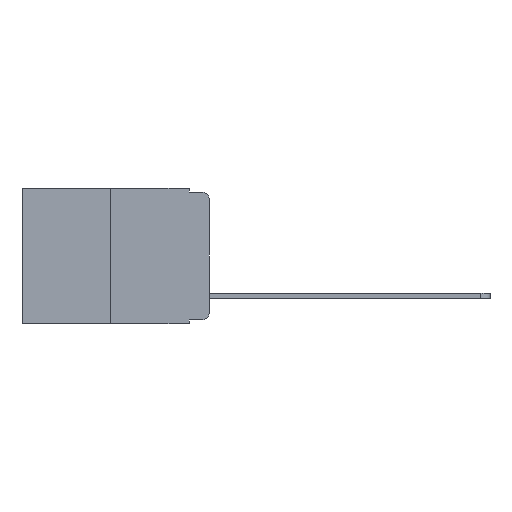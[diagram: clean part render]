
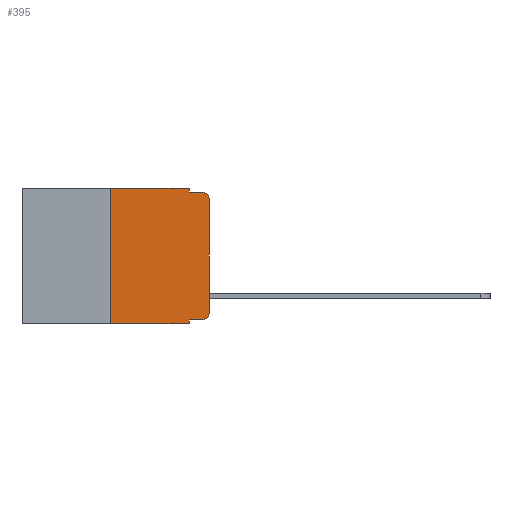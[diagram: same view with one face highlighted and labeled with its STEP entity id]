
A CAD part, left-side view. The second image highlights one B-rep face of the part: STEP entity #395.
In plain terms, the highlighted planar face has unit normal (-1, 0, 0).
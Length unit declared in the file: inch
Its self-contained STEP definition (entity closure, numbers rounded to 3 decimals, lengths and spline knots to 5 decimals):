
#41 = VERTEX_POINT ( 'NONE', #4234 ) ;
#271 = EDGE_CURVE ( 'NONE', #1706, #6711, #9293, .T. ) ;
#337 = VERTEX_POINT ( 'NONE', #8709 ) ;
#395 = ADVANCED_FACE ( 'NONE', ( #1490 ), #6747, .F. ) ;
#448 = VECTOR ( 'NONE', #8648, 39.37008 ) ;
#515 = DIRECTION ( 'NONE',  ( 0., -1., 0. ) ) ;
#679 = ORIENTED_EDGE ( 'NONE', *, *, #7900, .F. ) ;
#728 = LINE ( 'NONE', #1204, #448 ) ;
#745 = VECTOR ( 'NONE', #4934, 39.37008 ) ;
#969 = ORIENTED_EDGE ( 'NONE', *, *, #10487, .T. ) ;
#1012 = CARTESIAN_POINT ( 'NONE',  ( 0., 0.02, -0.333 ) ) ;
#1031 = EDGE_LOOP ( 'NONE', ( #1630, #4977, #679, #3099, #3904, #8712, #969, #8114, #4585, #9305 ) ) ;
#1162 = CARTESIAN_POINT ( 'NONE',  ( 0., 0., -0.313 ) ) ;
#1204 = CARTESIAN_POINT ( 'NONE',  ( 0., 0.051, -0.01 ) ) ;
#1225 = AXIS2_PLACEMENT_3D ( 'NONE', #5626, #6207, #6199 ) ;
#1490 = FACE_OUTER_BOUND ( 'NONE', #1031, .T. ) ;
#1497 = LINE ( 'NONE', #6130, #9902 ) ;
#1523 = EDGE_CURVE ( 'NONE', #337, #6897, #10321, .T. ) ;
#1630 = ORIENTED_EDGE ( 'NONE', *, *, #271, .T. ) ;
#1706 = VERTEX_POINT ( 'NONE', #1162 ) ;
#1831 = VERTEX_POINT ( 'NONE', #6097 ) ;
#1940 = VERTEX_POINT ( 'NONE', #7417 ) ;
#2019 = EDGE_CURVE ( 'NONE', #6711, #41, #8284, .T. ) ;
#2020 = EDGE_CURVE ( 'NONE', #2855, #1706, #10310, .T. ) ;
#2799 = DIRECTION ( 'NONE',  ( 0., -1., 0. ) ) ;
#2855 = VERTEX_POINT ( 'NONE', #1012 ) ;
#2981 = EDGE_CURVE ( 'NONE', #6897, #1940, #7904, .T. ) ;
#3023 = LINE ( 'NONE', #10417, #745 ) ;
#3099 = ORIENTED_EDGE ( 'NONE', *, *, #5181, .F. ) ;
#3163 = CARTESIAN_POINT ( 'NONE',  ( 0., 0.051, -0.01 ) ) ;
#3527 = AXIS2_PLACEMENT_3D ( 'NONE', #3577, #4171, #7919 ) ;
#3577 = CARTESIAN_POINT ( 'NONE',  ( 0., 0.02, -0.03 ) ) ;
#3611 = CARTESIAN_POINT ( 'NONE',  ( 0., 0.473, 0. ) ) ;
#3904 = ORIENTED_EDGE ( 'NONE', *, *, #2981, .F. ) ;
#3983 = VECTOR ( 'NONE', #7797, 39.37008 ) ;
#4027 = VECTOR ( 'NONE', #2799, 39.37008 ) ;
#4171 = DIRECTION ( 'NONE',  ( -1., 0., 0. ) ) ;
#4234 = CARTESIAN_POINT ( 'NONE',  ( 0., 0.02, -0.01 ) ) ;
#4266 = DIRECTION ( 'NONE',  ( 0., -1., 0. ) ) ;
#4585 = ORIENTED_EDGE ( 'NONE', *, *, #5970, .T. ) ;
#4663 = AXIS2_PLACEMENT_3D ( 'NONE', #7662, #8071, #6866 ) ;
#4756 = CARTESIAN_POINT ( 'NONE',  ( 0., 0.051, -0.333 ) ) ;
#4934 = DIRECTION ( 'NONE',  ( 0., 0., -1. ) ) ;
#4977 = ORIENTED_EDGE ( 'NONE', *, *, #2019, .T. ) ;
#5181 = EDGE_CURVE ( 'NONE', #1940, #9595, #1497, .T. ) ;
#5460 = DIRECTION ( 'NONE',  ( 0., 0., -1. ) ) ;
#5626 = CARTESIAN_POINT ( 'NONE',  ( 0., 0.473, 0. ) ) ;
#5808 = VECTOR ( 'NONE', #515, 39.37008 ) ;
#5970 = EDGE_CURVE ( 'NONE', #6853, #2855, #6730, .T. ) ;
#6097 = CARTESIAN_POINT ( 'NONE',  ( 0., 0.051, -0.343 ) ) ;
#6130 = CARTESIAN_POINT ( 'NONE',  ( 0., 0.051, 0. ) ) ;
#6199 = DIRECTION ( 'NONE',  ( 0., 0., -1. ) ) ;
#6207 = DIRECTION ( 'NONE',  ( 1., 0., 0. ) ) ;
#6240 = LINE ( 'NONE', #10011, #4027 ) ;
#6711 = VERTEX_POINT ( 'NONE', #7780 ) ;
#6730 = LINE ( 'NONE', #9470, #10590 ) ;
#6747 = PLANE ( 'NONE',  #1225 ) ;
#6853 = VERTEX_POINT ( 'NONE', #4756 ) ;
#6866 = DIRECTION ( 'NONE',  ( 0., 0., -1. ) ) ;
#6897 = VERTEX_POINT ( 'NONE', #8162 ) ;
#7417 = CARTESIAN_POINT ( 'NONE',  ( 0., 0.051, 0. ) ) ;
#7459 = EDGE_CURVE ( 'NONE', #6853, #1831, #3023, .T. ) ;
#7662 = CARTESIAN_POINT ( 'NONE',  ( 0., 0.02, -0.313 ) ) ;
#7780 = CARTESIAN_POINT ( 'NONE',  ( 0., 0., -0.03 ) ) ;
#7797 = DIRECTION ( 'NONE',  ( 0., 0., 1. ) ) ;
#7900 = EDGE_CURVE ( 'NONE', #9595, #41, #728, .T. ) ;
#7904 = LINE ( 'NONE', #3611, #5808 ) ;
#7919 = DIRECTION ( 'NONE',  ( 0., 0., -1. ) ) ;
#7931 = CARTESIAN_POINT ( 'NONE',  ( 0., 0., 0. ) ) ;
#7943 = DIRECTION ( 'NONE',  ( 0., 0., 1. ) ) ;
#8071 = DIRECTION ( 'NONE',  ( -1., 0., 0. ) ) ;
#8114 = ORIENTED_EDGE ( 'NONE', *, *, #7459, .F. ) ;
#8162 = CARTESIAN_POINT ( 'NONE',  ( 0., 0.25, 0. ) ) ;
#8284 = CIRCLE ( 'NONE', #3527, 0.02 ) ;
#8648 = DIRECTION ( 'NONE',  ( 0., -1., 0. ) ) ;
#8709 = CARTESIAN_POINT ( 'NONE',  ( 0., 0.25, -0.343 ) ) ;
#8712 = ORIENTED_EDGE ( 'NONE', *, *, #1523, .F. ) ;
#8828 = VECTOR ( 'NONE', #7943, 39.37008 ) ;
#9293 = LINE ( 'NONE', #7931, #8828 ) ;
#9305 = ORIENTED_EDGE ( 'NONE', *, *, #2020, .T. ) ;
#9470 = CARTESIAN_POINT ( 'NONE',  ( 0., 0.051, -0.333 ) ) ;
#9595 = VERTEX_POINT ( 'NONE', #3163 ) ;
#9902 = VECTOR ( 'NONE', #5460, 39.37008 ) ;
#10010 = CARTESIAN_POINT ( 'NONE',  ( 0., 0.25, 0. ) ) ;
#10011 = CARTESIAN_POINT ( 'NONE',  ( 0., 0.473, -0.343 ) ) ;
#10310 = CIRCLE ( 'NONE', #4663, 0.02 ) ;
#10321 = LINE ( 'NONE', #10010, #3983 ) ;
#10417 = CARTESIAN_POINT ( 'NONE',  ( 0., 0.051, 0. ) ) ;
#10487 = EDGE_CURVE ( 'NONE', #337, #1831, #6240, .T. ) ;
#10590 = VECTOR ( 'NONE', #4266, 39.37008 ) ;
